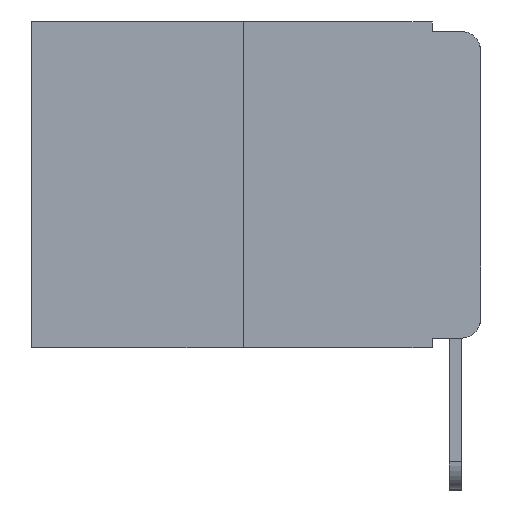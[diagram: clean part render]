
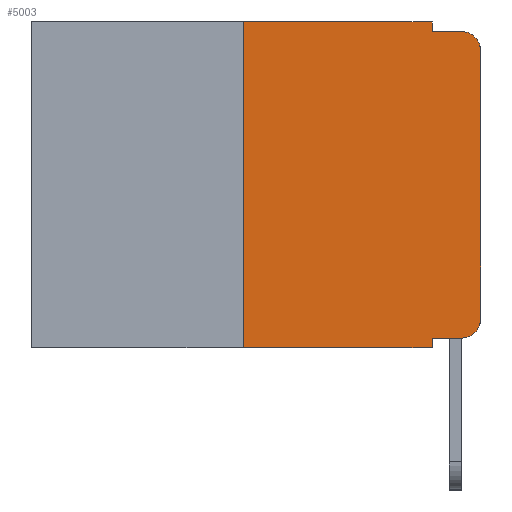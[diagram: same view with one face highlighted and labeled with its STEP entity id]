
A CAD part, left-side view. The second image highlights one B-rep face of the part: STEP entity #5003.
In plain terms, the highlighted planar face has unit normal (-1, 0, 0).
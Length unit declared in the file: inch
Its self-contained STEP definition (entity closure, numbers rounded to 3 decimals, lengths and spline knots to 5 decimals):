
#154 = EDGE_CURVE ( 'NONE', #8916, #8654, #4516, .T. ) ;
#181 = AXIS2_PLACEMENT_3D ( 'NONE', #754, #864, #2080 ) ;
#207 = CARTESIAN_POINT ( 'NONE',  ( 0., 0.02, -0.01 ) ) ;
#244 = DIRECTION ( 'NONE',  ( 0., 0., -1. ) ) ;
#265 = DIRECTION ( 'NONE',  ( 0., 0., 1. ) ) ;
#501 = ORIENTED_EDGE ( 'NONE', *, *, #3579, .F. ) ;
#754 = CARTESIAN_POINT ( 'NONE',  ( 0., 0.02, -0.03 ) ) ;
#864 = DIRECTION ( 'NONE',  ( -1., 0., 0. ) ) ;
#1392 = VERTEX_POINT ( 'NONE', #8805 ) ;
#1426 = DIRECTION ( 'NONE',  ( 0., 0., -1. ) ) ;
#1447 = DIRECTION ( 'NONE',  ( -1., 0., 0. ) ) ;
#1477 = CARTESIAN_POINT ( 'NONE',  ( 0., 0.02, -0.313 ) ) ;
#1497 = ORIENTED_EDGE ( 'NONE', *, *, #3484, .T. ) ;
#1518 = PLANE ( 'NONE',  #5905 ) ;
#1661 = DIRECTION ( 'NONE',  ( 0., 0., -1. ) ) ;
#1673 = DIRECTION ( 'NONE',  ( 1., 0., 0. ) ) ;
#2031 = EDGE_CURVE ( 'NONE', #11648, #9177, #8446, .T. ) ;
#2080 = DIRECTION ( 'NONE',  ( 0., 0., -1. ) ) ;
#2092 = VERTEX_POINT ( 'NONE', #2631 ) ;
#2149 = CARTESIAN_POINT ( 'NONE',  ( 0., 0.25, 0. ) ) ;
#2379 = VECTOR ( 'NONE', #4900, 39.37008 ) ;
#2631 = CARTESIAN_POINT ( 'NONE',  ( 0., 0.02, -0.333 ) ) ;
#2726 = DIRECTION ( 'NONE',  ( 0., 0., -1. ) ) ;
#2729 = LINE ( 'NONE', #6038, #2379 ) ;
#2855 = ORIENTED_EDGE ( 'NONE', *, *, #3688, .F. ) ;
#2907 = VECTOR ( 'NONE', #12746, 39.37008 ) ;
#3074 = VECTOR ( 'NONE', #265, 39.37008 ) ;
#3198 = ORIENTED_EDGE ( 'NONE', *, *, #3787, .T. ) ;
#3420 = VECTOR ( 'NONE', #1426, 39.37008 ) ;
#3484 = EDGE_CURVE ( 'NONE', #9036, #12327, #8858, .T. ) ;
#3513 = EDGE_CURVE ( 'NONE', #12327, #6931, #12664, .T. ) ;
#3579 = EDGE_CURVE ( 'NONE', #8779, #6931, #11867, .T. ) ;
#3688 = EDGE_CURVE ( 'NONE', #8654, #8779, #6666, .T. ) ;
#3745 = EDGE_CURVE ( 'NONE', #11648, #8916, #6364, .T. ) ;
#3764 = EDGE_CURVE ( 'NONE', #1392, #9177, #6040, .T. ) ;
#3787 = EDGE_CURVE ( 'NONE', #1392, #2092, #2729, .T. ) ;
#3814 = EDGE_CURVE ( 'NONE', #2092, #9036, #7763, .T. ) ;
#4516 = LINE ( 'NONE', #7060, #11367 ) ;
#4737 = DIRECTION ( 'NONE',  ( 0., -1., 0. ) ) ;
#4845 = FACE_OUTER_BOUND ( 'NONE', #9872, .T. ) ;
#4900 = DIRECTION ( 'NONE',  ( 0., -1., 0. ) ) ;
#5003 = ADVANCED_FACE ( 'NONE', ( #4845 ), #1518, .F. ) ;
#5497 = ORIENTED_EDGE ( 'NONE', *, *, #3745, .F. ) ;
#5703 = CARTESIAN_POINT ( 'NONE',  ( 0., 0.473, -0.343 ) ) ;
#5751 = DIRECTION ( 'NONE',  ( 0., -1., 0. ) ) ;
#5905 = AXIS2_PLACEMENT_3D ( 'NONE', #9305, #1673, #2726 ) ;
#6038 = CARTESIAN_POINT ( 'NONE',  ( 0., 0.051, -0.333 ) ) ;
#6040 = LINE ( 'NONE', #12723, #12786 ) ;
#6364 = LINE ( 'NONE', #2149, #3074 ) ;
#6666 = LINE ( 'NONE', #9260, #3420 ) ;
#6931 = VERTEX_POINT ( 'NONE', #207 ) ;
#7060 = CARTESIAN_POINT ( 'NONE',  ( 0., 0.473, 0. ) ) ;
#7138 = DIRECTION ( 'NONE',  ( 0., -1., 0. ) ) ;
#7149 = AXIS2_PLACEMENT_3D ( 'NONE', #1477, #1447, #1661 ) ;
#7200 = ORIENTED_EDGE ( 'NONE', *, *, #3513, .T. ) ;
#7597 = VECTOR ( 'NONE', #7138, 39.37008 ) ;
#7763 = CIRCLE ( 'NONE', #7149, 0.02 ) ;
#7778 = CARTESIAN_POINT ( 'NONE',  ( 0., 0.051, 0. ) ) ;
#7996 = ORIENTED_EDGE ( 'NONE', *, *, #154, .F. ) ;
#8429 = CARTESIAN_POINT ( 'NONE',  ( 0., 0., -0.313 ) ) ;
#8446 = LINE ( 'NONE', #5703, #12560 ) ;
#8486 = CARTESIAN_POINT ( 'NONE',  ( 0., 0.25, -0.343 ) ) ;
#8532 = CARTESIAN_POINT ( 'NONE',  ( 0., 0.051, -0.01 ) ) ;
#8596 = CARTESIAN_POINT ( 'NONE',  ( 0., 0.051, -0.343 ) ) ;
#8654 = VERTEX_POINT ( 'NONE', #7778 ) ;
#8779 = VERTEX_POINT ( 'NONE', #10706 ) ;
#8805 = CARTESIAN_POINT ( 'NONE',  ( 0., 0.051, -0.333 ) ) ;
#8858 = LINE ( 'NONE', #12173, #2907 ) ;
#8916 = VERTEX_POINT ( 'NONE', #11023 ) ;
#9036 = VERTEX_POINT ( 'NONE', #8429 ) ;
#9177 = VERTEX_POINT ( 'NONE', #8596 ) ;
#9260 = CARTESIAN_POINT ( 'NONE',  ( 0., 0.051, 0. ) ) ;
#9305 = CARTESIAN_POINT ( 'NONE',  ( 0., 0.473, 0. ) ) ;
#9630 = ORIENTED_EDGE ( 'NONE', *, *, #3764, .F. ) ;
#9872 = EDGE_LOOP ( 'NONE', ( #1497, #7200, #501, #2855, #7996, #5497, #11415, #9630, #3198, #10553 ) ) ;
#10553 = ORIENTED_EDGE ( 'NONE', *, *, #3814, .T. ) ;
#10706 = CARTESIAN_POINT ( 'NONE',  ( 0., 0.051, -0.01 ) ) ;
#11023 = CARTESIAN_POINT ( 'NONE',  ( 0., 0.25, 0. ) ) ;
#11367 = VECTOR ( 'NONE', #5751, 39.37008 ) ;
#11415 = ORIENTED_EDGE ( 'NONE', *, *, #2031, .T. ) ;
#11588 = CARTESIAN_POINT ( 'NONE',  ( 0., 0., -0.03 ) ) ;
#11648 = VERTEX_POINT ( 'NONE', #8486 ) ;
#11867 = LINE ( 'NONE', #8532, #7597 ) ;
#12173 = CARTESIAN_POINT ( 'NONE',  ( 0., 0., 0. ) ) ;
#12327 = VERTEX_POINT ( 'NONE', #11588 ) ;
#12560 = VECTOR ( 'NONE', #4737, 39.37008 ) ;
#12664 = CIRCLE ( 'NONE', #181, 0.02 ) ;
#12723 = CARTESIAN_POINT ( 'NONE',  ( 0., 0.051, 0. ) ) ;
#12746 = DIRECTION ( 'NONE',  ( 0., 0., 1. ) ) ;
#12786 = VECTOR ( 'NONE', #244, 39.37008 ) ;
